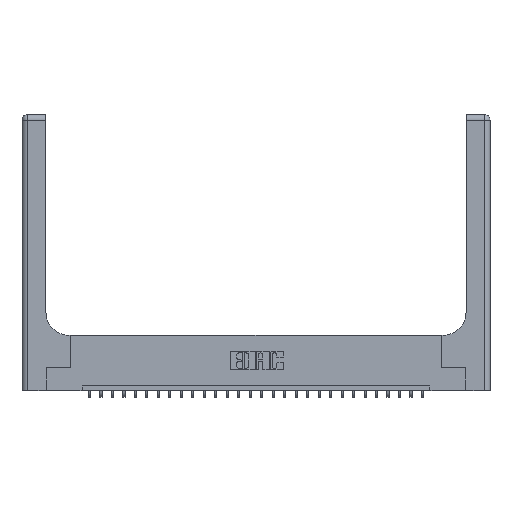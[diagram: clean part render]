
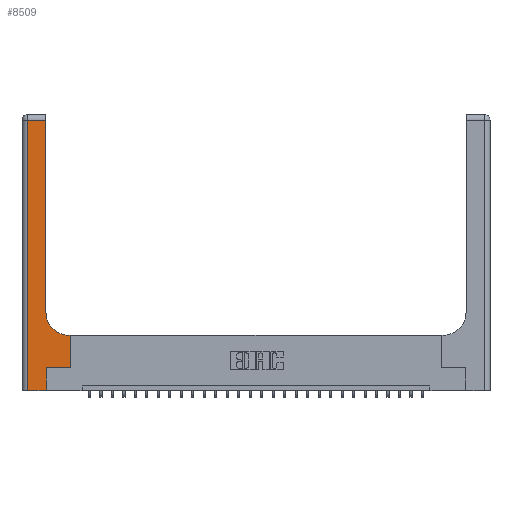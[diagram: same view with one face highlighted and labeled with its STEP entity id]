
A CAD part, top view. The second image highlights one B-rep face of the part: STEP entity #8509.
In plain terms, the highlighted planar face has unit normal (0, 0, 1).
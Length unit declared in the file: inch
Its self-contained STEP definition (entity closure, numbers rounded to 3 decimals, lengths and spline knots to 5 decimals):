
#52 = VERTEX_POINT ( 'NONE', #21927 ) ;
#100 = EDGE_CURVE ( 'NONE', #20524, #10768, #13193, .T. ) ;
#158 = VECTOR ( 'NONE', #22138, 39.37008 ) ;
#1412 = DIRECTION ( 'NONE',  ( 0., -1., 0. ) ) ;
#2714 = ORIENTED_EDGE ( 'NONE', *, *, #22908, .T. ) ;
#3003 = DIRECTION ( 'NONE',  ( -1., 0., 0. ) ) ;
#4124 = CARTESIAN_POINT ( 'NONE',  ( 0.26, 3., 0.37 ) ) ;
#4174 = VERTEX_POINT ( 'NONE', #19271 ) ;
#4178 = DIRECTION ( 'NONE',  ( 0., 1., 0. ) ) ;
#4499 = EDGE_CURVE ( 'NONE', #15741, #18250, #23922, .T. ) ;
#5399 = DIRECTION ( 'NONE',  ( 0., 0., -1. ) ) ;
#5584 = ORIENTED_EDGE ( 'NONE', *, *, #4499, .T. ) ;
#6691 = CARTESIAN_POINT ( 'NONE',  ( 0., 3., 0.37 ) ) ;
#6810 = VECTOR ( 'NONE', #3003, 39.37008 ) ;
#7312 = VECTOR ( 'NONE', #25279, 39.37008 ) ;
#7391 = CARTESIAN_POINT ( 'NONE',  ( 0.06, 3., 0.37 ) ) ;
#7852 = LINE ( 'NONE', #19087, #18334 ) ;
#8369 = CARTESIAN_POINT ( 'NONE',  ( 0.26, 0.6, 0.37 ) ) ;
#8509 = ADVANCED_FACE ( 'NONE', ( #15530 ), #14552, .F. ) ;
#9406 = CARTESIAN_POINT ( 'NONE',  ( 0.26, 2.94, 0.37 ) ) ;
#9557 = CARTESIAN_POINT ( 'NONE',  ( 0.528, 0.6, 0.37 ) ) ;
#9597 = CARTESIAN_POINT ( 'NONE',  ( 0.51, 0.6, 0.37 ) ) ;
#10529 = ORIENTED_EDGE ( 'NONE', *, *, #11210, .T. ) ;
#10649 = DIRECTION ( 'NONE',  ( -1., 0., 0. ) ) ;
#10696 = AXIS2_PLACEMENT_3D ( 'NONE', #17226, #5399, #19180 ) ;
#10768 = VERTEX_POINT ( 'NONE', #19935 ) ;
#11210 = EDGE_CURVE ( 'NONE', #10768, #14826, #21930, .T. ) ;
#11481 = VECTOR ( 'NONE', #4178, 39.37008 ) ;
#11933 = ORIENTED_EDGE ( 'NONE', *, *, #16188, .T. ) ;
#11936 = VERTEX_POINT ( 'NONE', #9406 ) ;
#12451 = EDGE_CURVE ( 'NONE', #23670, #52, #15766, .T. ) ;
#12703 = LINE ( 'NONE', #18700, #6810 ) ;
#13193 = LINE ( 'NONE', #25194, #7312 ) ;
#14126 = ORIENTED_EDGE ( 'NONE', *, *, #21498, .T. ) ;
#14364 = LINE ( 'NONE', #7391, #24776 ) ;
#14453 = DIRECTION ( 'NONE',  ( 1., 0., 0. ) ) ;
#14552 = PLANE ( 'NONE',  #17919 ) ;
#14826 = VERTEX_POINT ( 'NONE', #9557 ) ;
#15141 = CARTESIAN_POINT ( 'NONE',  ( 0.06, 0., 0.37 ) ) ;
#15165 = DIRECTION ( 'NONE',  ( 0., 1., 0. ) ) ;
#15271 = ORIENTED_EDGE ( 'NONE', *, *, #19648, .T. ) ;
#15530 = FACE_OUTER_BOUND ( 'NONE', #21121, .T. ) ;
#15741 = VERTEX_POINT ( 'NONE', #15141 ) ;
#15766 = CIRCLE ( 'NONE', #10696, 0.25 ) ;
#16188 = EDGE_CURVE ( 'NONE', #11936, #4174, #12703, .T. ) ;
#17226 = CARTESIAN_POINT ( 'NONE',  ( 0.51, 0.85, 0.37 ) ) ;
#17534 = ORIENTED_EDGE ( 'NONE', *, *, #22167, .T. ) ;
#17919 = AXIS2_PLACEMENT_3D ( 'NONE', #6691, #22430, #10649 ) ;
#17984 = DIRECTION ( 'NONE',  ( 0., 1., 0. ) ) ;
#18250 = VERTEX_POINT ( 'NONE', #22594 ) ;
#18334 = VECTOR ( 'NONE', #15165, 39.37008 ) ;
#18700 = CARTESIAN_POINT ( 'NONE',  ( 0., 2.94, 0.37 ) ) ;
#19087 = CARTESIAN_POINT ( 'NONE',  ( 0.265, 0., 0.37 ) ) ;
#19180 = DIRECTION ( 'NONE',  ( 1., 0., 0. ) ) ;
#19271 = CARTESIAN_POINT ( 'NONE',  ( 0.06, 2.94, 0.37 ) ) ;
#19648 = EDGE_CURVE ( 'NONE', #18250, #20524, #7852, .T. ) ;
#19935 = CARTESIAN_POINT ( 'NONE',  ( 0.528, 0.25, 0.37 ) ) ;
#20301 = CARTESIAN_POINT ( 'NONE',  ( 0., 0., 0.37 ) ) ;
#20306 = ORIENTED_EDGE ( 'NONE', *, *, #12451, .T. ) ;
#20524 = VERTEX_POINT ( 'NONE', #25020 ) ;
#20562 = LINE ( 'NONE', #8369, #158 ) ;
#20902 = VECTOR ( 'NONE', #17984, 39.37008 ) ;
#21121 = EDGE_LOOP ( 'NONE', ( #14126, #11933, #2714, #5584, #15271, #23487, #10529, #17534, #20306 ) ) ;
#21498 = EDGE_CURVE ( 'NONE', #52, #11936, #21504, .T. ) ;
#21504 = LINE ( 'NONE', #4124, #20902 ) ;
#21805 = CARTESIAN_POINT ( 'NONE',  ( 0.528, 0.25, 0.37 ) ) ;
#21927 = CARTESIAN_POINT ( 'NONE',  ( 0.26, 0.85, 0.37 ) ) ;
#21930 = LINE ( 'NONE', #21805, #11481 ) ;
#22116 = VECTOR ( 'NONE', #14453, 39.37008 ) ;
#22138 = DIRECTION ( 'NONE',  ( -1., 0., 0. ) ) ;
#22167 = EDGE_CURVE ( 'NONE', #14826, #23670, #20562, .T. ) ;
#22430 = DIRECTION ( 'NONE',  ( 0., 0., -1. ) ) ;
#22594 = CARTESIAN_POINT ( 'NONE',  ( 0.265, 0., 0.37 ) ) ;
#22908 = EDGE_CURVE ( 'NONE', #4174, #15741, #14364, .T. ) ;
#23487 = ORIENTED_EDGE ( 'NONE', *, *, #100, .T. ) ;
#23670 = VERTEX_POINT ( 'NONE', #9597 ) ;
#23922 = LINE ( 'NONE', #20301, #22116 ) ;
#24776 = VECTOR ( 'NONE', #1412, 39.37008 ) ;
#25020 = CARTESIAN_POINT ( 'NONE',  ( 0.265, 0.25, 0.37 ) ) ;
#25194 = CARTESIAN_POINT ( 'NONE',  ( 0.265, 0.25, 0.37 ) ) ;
#25279 = DIRECTION ( 'NONE',  ( 1., 0., 0. ) ) ;
